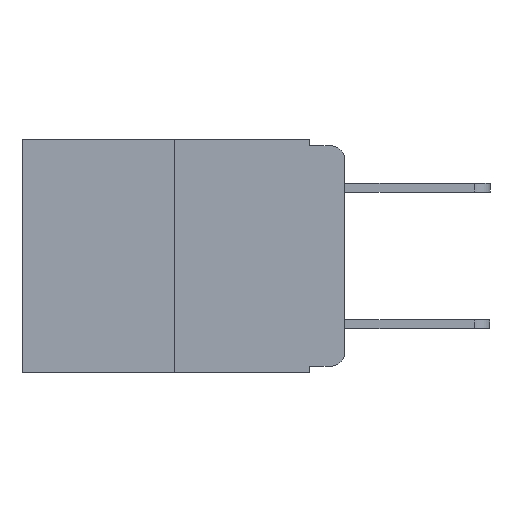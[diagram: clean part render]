
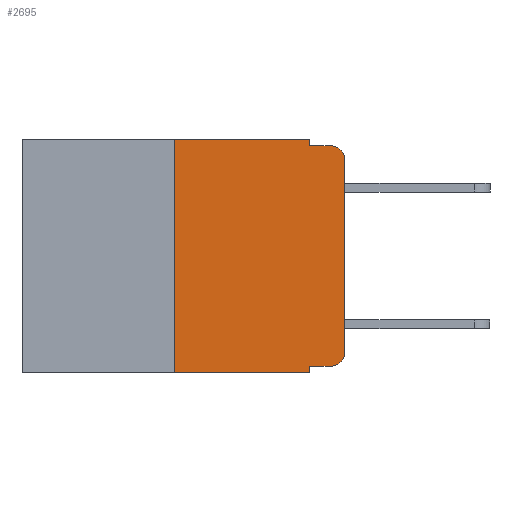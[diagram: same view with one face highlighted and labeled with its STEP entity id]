
A CAD part, left-side view. The second image highlights one B-rep face of the part: STEP entity #2695.
In plain terms, the highlighted planar face has unit normal (-1, 0, 0).
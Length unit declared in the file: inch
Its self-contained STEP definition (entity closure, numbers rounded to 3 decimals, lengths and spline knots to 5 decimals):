
#410 = CIRCLE ( 'NONE', #13939, 0.02 ) ;
#474 = VERTEX_POINT ( 'NONE', #16540 ) ;
#637 = DIRECTION ( 'NONE',  ( 0., 0., -1. ) ) ;
#976 = CARTESIAN_POINT ( 'NONE',  ( 0., 0., -0.03 ) ) ;
#1137 = VERTEX_POINT ( 'NONE', #15778 ) ;
#1521 = CARTESIAN_POINT ( 'NONE',  ( 0., 0., 0. ) ) ;
#1969 = EDGE_CURVE ( 'NONE', #3160, #9240, #16323, .T. ) ;
#2532 = CARTESIAN_POINT ( 'NONE',  ( 0., 0.051, -0.343 ) ) ;
#2582 = LINE ( 'NONE', #11421, #17844 ) ;
#2674 = CARTESIAN_POINT ( 'NONE',  ( 0., 0.051, 0. ) ) ;
#2695 = ADVANCED_FACE ( 'NONE', ( #5433 ), #15304, .F. ) ;
#2745 = VERTEX_POINT ( 'NONE', #16639 ) ;
#3160 = VERTEX_POINT ( 'NONE', #13465 ) ;
#3172 = DIRECTION ( 'NONE',  ( 0., 0., 1. ) ) ;
#3210 = EDGE_CURVE ( 'NONE', #474, #3771, #17078, .T. ) ;
#3771 = VERTEX_POINT ( 'NONE', #4889 ) ;
#4462 = DIRECTION ( 'NONE',  ( 0., 0., -1. ) ) ;
#4525 = DIRECTION ( 'NONE',  ( 1., 0., 0. ) ) ;
#4889 = CARTESIAN_POINT ( 'NONE',  ( 0., 0.02, -0.333 ) ) ;
#5433 = FACE_OUTER_BOUND ( 'NONE', #8473, .T. ) ;
#5475 = DIRECTION ( 'NONE',  ( 0., -1., 0. ) ) ;
#5842 = ORIENTED_EDGE ( 'NONE', *, *, #18785, .T. ) ;
#5911 = ORIENTED_EDGE ( 'NONE', *, *, #10274, .T. ) ;
#5989 = ORIENTED_EDGE ( 'NONE', *, *, #7214, .F. ) ;
#5991 = ORIENTED_EDGE ( 'NONE', *, *, #16832, .F. ) ;
#6056 = DIRECTION ( 'NONE',  ( 0., -1., 0. ) ) ;
#6165 = ORIENTED_EDGE ( 'NONE', *, *, #1969, .F. ) ;
#6186 = ORIENTED_EDGE ( 'NONE', *, *, #11727, .F. ) ;
#6223 = EDGE_CURVE ( 'NONE', #18196, #17620, #18457, .T. ) ;
#6313 = ORIENTED_EDGE ( 'NONE', *, *, #6223, .T. ) ;
#6333 = ORIENTED_EDGE ( 'NONE', *, *, #14505, .F. ) ;
#6357 = CARTESIAN_POINT ( 'NONE',  ( 0., 0.051, -0.01 ) ) ;
#6382 = VERTEX_POINT ( 'NONE', #976 ) ;
#6442 = CARTESIAN_POINT ( 'NONE',  ( 0., 0.051, 0. ) ) ;
#6486 = VECTOR ( 'NONE', #16201, 39.37008 ) ;
#6546 = EDGE_CURVE ( 'NONE', #3771, #10506, #410, .T. ) ;
#6583 = ORIENTED_EDGE ( 'NONE', *, *, #3210, .T. ) ;
#6682 = ORIENTED_EDGE ( 'NONE', *, *, #6546, .T. ) ;
#6976 = LINE ( 'NONE', #18714, #6486 ) ;
#7214 = EDGE_CURVE ( 'NONE', #2745, #1137, #8692, .T. ) ;
#7838 = LINE ( 'NONE', #6442, #18972 ) ;
#8269 = VECTOR ( 'NONE', #15604, 39.37008 ) ;
#8400 = CARTESIAN_POINT ( 'NONE',  ( 0., 0.051, -0.333 ) ) ;
#8473 = EDGE_LOOP ( 'NONE', ( #5842, #5911, #5989, #5991, #6165, #6186, #6313, #6333, #6583, #6682 ) ) ;
#8692 = LINE ( 'NONE', #6357, #12222 ) ;
#9224 = VECTOR ( 'NONE', #6056, 39.37008 ) ;
#9240 = VERTEX_POINT ( 'NONE', #2674 ) ;
#9377 = CARTESIAN_POINT ( 'NONE',  ( 0., 0., -0.313 ) ) ;
#9616 = DIRECTION ( 'NONE',  ( -1., 0., 0. ) ) ;
#10119 = CARTESIAN_POINT ( 'NONE',  ( 0., 0.25, -0.343 ) ) ;
#10274 = EDGE_CURVE ( 'NONE', #6382, #1137, #12752, .T. ) ;
#10422 = DIRECTION ( 'NONE',  ( -1., 0., 0. ) ) ;
#10506 = VERTEX_POINT ( 'NONE', #9377 ) ;
#11421 = CARTESIAN_POINT ( 'NONE',  ( 0., 0.25, 0. ) ) ;
#11727 = EDGE_CURVE ( 'NONE', #18196, #3160, #2582, .T. ) ;
#12139 = CARTESIAN_POINT ( 'NONE',  ( 0., 0.473, 0. ) ) ;
#12222 = VECTOR ( 'NONE', #17820, 39.37008 ) ;
#12231 = VECTOR ( 'NONE', #5475, 39.37008 ) ;
#12307 = CARTESIAN_POINT ( 'NONE',  ( 0., 0.473, 0. ) ) ;
#12752 = CIRCLE ( 'NONE', #17962, 0.02 ) ;
#13231 = AXIS2_PLACEMENT_3D ( 'NONE', #12307, #4525, #4462 ) ;
#13254 = VECTOR ( 'NONE', #3172, 39.37008 ) ;
#13465 = CARTESIAN_POINT ( 'NONE',  ( 0., 0.25, 0. ) ) ;
#13685 = LINE ( 'NONE', #1521, #13254 ) ;
#13939 = AXIS2_PLACEMENT_3D ( 'NONE', #17864, #9616, #19142 ) ;
#14505 = EDGE_CURVE ( 'NONE', #474, #17620, #7838, .T. ) ;
#15304 = PLANE ( 'NONE',  #13231 ) ;
#15604 = DIRECTION ( 'NONE',  ( 0., -1., 0. ) ) ;
#15623 = DIRECTION ( 'NONE',  ( 0., 0., 1. ) ) ;
#15778 = CARTESIAN_POINT ( 'NONE',  ( 0., 0.02, -0.01 ) ) ;
#15868 = CARTESIAN_POINT ( 'NONE',  ( 0., 0.473, -0.343 ) ) ;
#16201 = DIRECTION ( 'NONE',  ( 0., 0., -1. ) ) ;
#16323 = LINE ( 'NONE', #12139, #8269 ) ;
#16540 = CARTESIAN_POINT ( 'NONE',  ( 0., 0.051, -0.333 ) ) ;
#16639 = CARTESIAN_POINT ( 'NONE',  ( 0., 0.051, -0.01 ) ) ;
#16832 = EDGE_CURVE ( 'NONE', #9240, #2745, #6976, .T. ) ;
#17078 = LINE ( 'NONE', #8400, #9224 ) ;
#17620 = VERTEX_POINT ( 'NONE', #2532 ) ;
#17820 = DIRECTION ( 'NONE',  ( 0., -1., 0. ) ) ;
#17844 = VECTOR ( 'NONE', #15623, 39.37008 ) ;
#17864 = CARTESIAN_POINT ( 'NONE',  ( 0., 0.02, -0.313 ) ) ;
#17882 = DIRECTION ( 'NONE',  ( 0., 0., -1. ) ) ;
#17962 = AXIS2_PLACEMENT_3D ( 'NONE', #18519, #10422, #637 ) ;
#18196 = VERTEX_POINT ( 'NONE', #10119 ) ;
#18457 = LINE ( 'NONE', #15868, #12231 ) ;
#18519 = CARTESIAN_POINT ( 'NONE',  ( 0., 0.02, -0.03 ) ) ;
#18714 = CARTESIAN_POINT ( 'NONE',  ( 0., 0.051, 0. ) ) ;
#18785 = EDGE_CURVE ( 'NONE', #10506, #6382, #13685, .T. ) ;
#18972 = VECTOR ( 'NONE', #17882, 39.37008 ) ;
#19142 = DIRECTION ( 'NONE',  ( 0., 0., -1. ) ) ;
